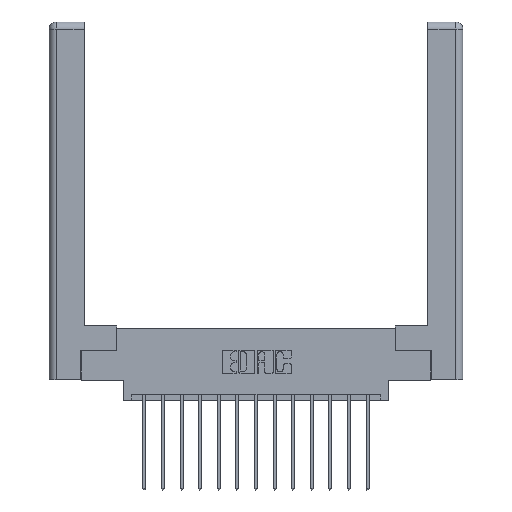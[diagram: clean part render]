
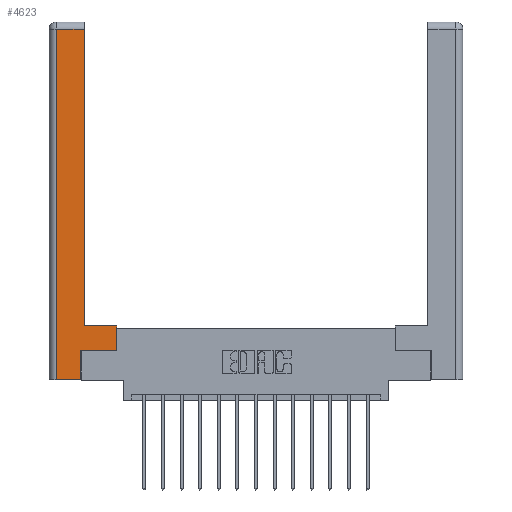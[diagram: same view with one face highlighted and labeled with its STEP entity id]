
A CAD part, top view. The second image highlights one B-rep face of the part: STEP entity #4623.
In plain terms, the highlighted planar face has unit normal (0, 0, 1).
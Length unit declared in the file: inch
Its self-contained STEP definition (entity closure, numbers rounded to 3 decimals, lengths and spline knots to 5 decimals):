
#143 = VECTOR ( 'NONE', #2542, 39.37008 ) ;
#327 = CARTESIAN_POINT ( 'NONE',  ( 0.295, 2.94, 0. ) ) ;
#455 = VERTEX_POINT ( 'NONE', #6798 ) ;
#790 = CARTESIAN_POINT ( 'NONE',  ( 0.565, 0.245, 0. ) ) ;
#916 = VERTEX_POINT ( 'NONE', #5087 ) ;
#1211 = LINE ( 'NONE', #790, #10678 ) ;
#1708 = CARTESIAN_POINT ( 'NONE',  ( 0.265, 0., 0. ) ) ;
#2105 = DIRECTION ( 'NONE',  ( 1., 0., 0. ) ) ;
#2542 = DIRECTION ( 'NONE',  ( 0., 1., 0. ) ) ;
#2902 = CARTESIAN_POINT ( 'NONE',  ( 0.295, 0.45, 0. ) ) ;
#2953 = VECTOR ( 'NONE', #10506, 39.37008 ) ;
#3751 = LINE ( 'NONE', #6320, #2953 ) ;
#4006 = VERTEX_POINT ( 'NONE', #10313 ) ;
#4375 = CARTESIAN_POINT ( 'NONE',  ( 0.565, 0.45, 0. ) ) ;
#4623 = ADVANCED_FACE ( 'NONE', ( #9566 ), #6666, .F. ) ;
#4913 = EDGE_CURVE ( 'NONE', #16441, #4006, #15344, .T. ) ;
#4947 = ORIENTED_EDGE ( 'NONE', *, *, #15473, .T. ) ;
#5087 = CARTESIAN_POINT ( 'NONE',  ( 0.265, 0.245, 0. ) ) ;
#5653 = VECTOR ( 'NONE', #6148, 39.37008 ) ;
#6032 = LINE ( 'NONE', #13945, #10047 ) ;
#6148 = DIRECTION ( 'NONE',  ( -1., 0., 0. ) ) ;
#6320 = CARTESIAN_POINT ( 'NONE',  ( 0.295, 3., 0. ) ) ;
#6499 = DIRECTION ( 'NONE',  ( 0., 0., -1. ) ) ;
#6665 = EDGE_CURVE ( 'NONE', #916, #16441, #1211, .T. ) ;
#6666 = PLANE ( 'NONE',  #13867 ) ;
#6731 = VERTEX_POINT ( 'NONE', #10207 ) ;
#6798 = CARTESIAN_POINT ( 'NONE',  ( 0.0615, 0., 0. ) ) ;
#7101 = EDGE_CURVE ( 'NONE', #4006, #12927, #13472, .T. ) ;
#7201 = ORIENTED_EDGE ( 'NONE', *, *, #14837, .T. ) ;
#7218 = ORIENTED_EDGE ( 'NONE', *, *, #14295, .T. ) ;
#7474 = DIRECTION ( 'NONE',  ( 1., 0., 0. ) ) ;
#7540 = CARTESIAN_POINT ( 'NONE',  ( 0.265, 0.245, 0. ) ) ;
#7599 = VECTOR ( 'NONE', #7791, 39.37008 ) ;
#7791 = DIRECTION ( 'NONE',  ( 0., -1., 0. ) ) ;
#8029 = DIRECTION ( 'NONE',  ( 0., 1., 0. ) ) ;
#8818 = CARTESIAN_POINT ( 'NONE',  ( 0.265, 0., 0. ) ) ;
#9140 = DIRECTION ( 'NONE',  ( -1., 0., 0. ) ) ;
#9566 = FACE_OUTER_BOUND ( 'NONE', #13764, .T. ) ;
#9719 = CARTESIAN_POINT ( 'NONE',  ( 0.565, 0.245, 0. ) ) ;
#10047 = VECTOR ( 'NONE', #12650, 39.37008 ) ;
#10207 = CARTESIAN_POINT ( 'NONE',  ( 0.0615, 2.94, 0. ) ) ;
#10313 = CARTESIAN_POINT ( 'NONE',  ( 0.565, 0.45, 0. ) ) ;
#10413 = LINE ( 'NONE', #7540, #143 ) ;
#10506 = DIRECTION ( 'NONE',  ( 0., 1., 0. ) ) ;
#10554 = VECTOR ( 'NONE', #8029, 39.37008 ) ;
#10678 = VECTOR ( 'NONE', #2105, 39.37008 ) ;
#11069 = CARTESIAN_POINT ( 'NONE',  ( 0.295, 0.45, 0. ) ) ;
#11403 = CARTESIAN_POINT ( 'NONE',  ( 0.0615, 0., 0. ) ) ;
#11425 = VECTOR ( 'NONE', #7474, 39.37008 ) ;
#11526 = ORIENTED_EDGE ( 'NONE', *, *, #13126, .T. ) ;
#11815 = CARTESIAN_POINT ( 'NONE',  ( 0., 0., 0. ) ) ;
#12177 = VERTEX_POINT ( 'NONE', #327 ) ;
#12650 = DIRECTION ( 'NONE',  ( -1., 0., 0. ) ) ;
#12651 = ORIENTED_EDGE ( 'NONE', *, *, #6665, .T. ) ;
#12927 = VERTEX_POINT ( 'NONE', #2902 ) ;
#13126 = EDGE_CURVE ( 'NONE', #12177, #6731, #6032, .T. ) ;
#13472 = LINE ( 'NONE', #11069, #5653 ) ;
#13683 = ORIENTED_EDGE ( 'NONE', *, *, #14192, .T. ) ;
#13764 = EDGE_LOOP ( 'NONE', ( #7201, #11526, #4947, #13683, #7218, #12651, #15442, #15087 ) ) ;
#13806 = VERTEX_POINT ( 'NONE', #1708 ) ;
#13867 = AXIS2_PLACEMENT_3D ( 'NONE', #11815, #6499, #9140 ) ;
#13945 = CARTESIAN_POINT ( 'NONE',  ( 0.0615, 2.94, 0. ) ) ;
#14192 = EDGE_CURVE ( 'NONE', #455, #13806, #16411, .T. ) ;
#14295 = EDGE_CURVE ( 'NONE', #13806, #916, #10413, .T. ) ;
#14837 = EDGE_CURVE ( 'NONE', #12927, #12177, #3751, .T. ) ;
#15087 = ORIENTED_EDGE ( 'NONE', *, *, #7101, .T. ) ;
#15344 = LINE ( 'NONE', #4375, #10554 ) ;
#15442 = ORIENTED_EDGE ( 'NONE', *, *, #4913, .T. ) ;
#15473 = EDGE_CURVE ( 'NONE', #6731, #455, #15934, .T. ) ;
#15934 = LINE ( 'NONE', #11403, #7599 ) ;
#16411 = LINE ( 'NONE', #8818, #11425 ) ;
#16441 = VERTEX_POINT ( 'NONE', #9719 ) ;
